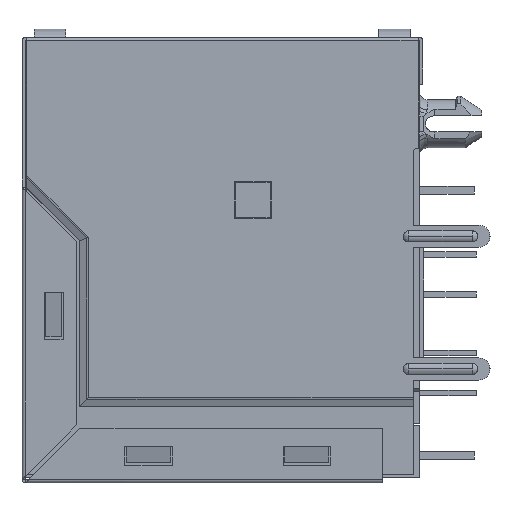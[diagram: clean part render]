
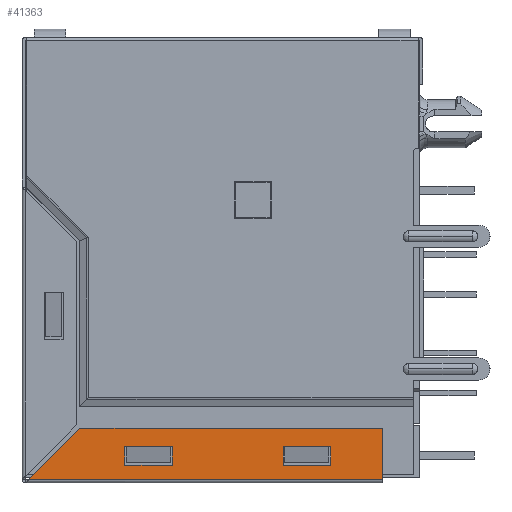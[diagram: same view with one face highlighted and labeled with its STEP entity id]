
A CAD part, left-side view. The second image highlights one B-rep face of the part: STEP entity #41363.
In plain terms, the highlighted planar face has unit normal (-1, 0, 0).
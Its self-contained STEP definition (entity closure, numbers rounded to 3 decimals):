
#149 = EDGE_CURVE ( 'NONE', #71271, #63621, #42202, .T. ) ;
#199 = EDGE_CURVE ( 'NONE', #31274, #15302, #2112, .T. ) ;
#1811 = EDGE_LOOP ( 'NONE', ( #43591, #2612, #13545, #4547 ) ) ;
#2112 = B_SPLINE_CURVE_WITH_KNOTS ( 'NONE', 1,
 ( #37321, #13007 ),
 .UNSPECIFIED., .F., .F.,
 ( 2, 2 ),
 ( 0., 1. ),
 .UNSPECIFIED. ) ;
#2612 = ORIENTED_EDGE ( 'NONE', *, *, #149, .T. ) ;
#3818 = CARTESIAN_POINT ( 'NONE',  ( -31.88, 6.165, -25.58 ) ) ;
#4150 = CARTESIAN_POINT ( 'NONE',  ( -31.88, 3.165, -25.58 ) ) ;
#4243 = CARTESIAN_POINT ( 'NONE',  ( -31.88, 6.165, -26.78 ) ) ;
#4261 = B_SPLINE_CURVE_WITH_KNOTS ( 'NONE', 1,
 ( #71911, #40936 ),
 .UNSPECIFIED., .F., .F.,
 ( 2, 2 ),
 ( 0., 1. ),
 .UNSPECIFIED. ) ;
#4446 = B_SPLINE_CURVE_WITH_KNOTS ( 'NONE', 1,
 ( #66529, #36102 ),
 .UNSPECIFIED., .F., .F.,
 ( 2, 2 ),
 ( 0., 1. ),
 .UNSPECIFIED. ) ;
#4547 = ORIENTED_EDGE ( 'NONE', *, *, #18581, .T. ) ;
#4903 = VECTOR ( 'NONE', #34564, 1000. ) ;
#9027 = CARTESIAN_POINT ( 'NONE',  ( -31.88, 9.005, -24.43 ) ) ;
#9712 = CARTESIAN_POINT ( 'NONE',  ( -31.88, 3.165, -26.78 ) ) ;
#10594 = EDGE_LOOP ( 'NONE', ( #33533, #55277, #71674, #60568 ) ) ;
#11064 = ORIENTED_EDGE ( 'NONE', *, *, #18309, .F. ) ;
#12041 = CARTESIAN_POINT ( 'NONE',  ( -31.88, 9.005, -24.43 ) ) ;
#12898 = CARTESIAN_POINT ( 'NONE',  ( -31.88, 6.165, -26.78 ) ) ;
#13007 = CARTESIAN_POINT ( 'NONE',  ( -31.88, 6.165, -25.58 ) ) ;
#13483 = VERTEX_POINT ( 'NONE', #12041 ) ;
#13545 = ORIENTED_EDGE ( 'NONE', *, *, #63434, .T. ) ;
#15302 = VERTEX_POINT ( 'NONE', #42465 ) ;
#15619 = CARTESIAN_POINT ( 'NONE',  ( -31.88, 1.055, -27.67 ) ) ;
#18309 = EDGE_CURVE ( 'NONE', #62407, #21727, #28934, .T. ) ;
#18581 = EDGE_CURVE ( 'NONE', #70747, #31402, #37221, .T. ) ;
#19591 = ORIENTED_EDGE ( 'NONE', *, *, #33564, .T. ) ;
#19681 = EDGE_CURVE ( 'NONE', #13483, #41862, #59765, .T. ) ;
#20091 = CARTESIAN_POINT ( 'NONE',  ( -31.88, -10.135, -24.43 ) ) ;
#21066 = CARTESIAN_POINT ( 'NONE',  ( -31.88, 12.245, -27.67 ) ) ;
#21727 = VERTEX_POINT ( 'NONE', #22345 ) ;
#22345 = CARTESIAN_POINT ( 'NONE',  ( -31.88, -10.135, -27.67 ) ) ;
#22449 = VERTEX_POINT ( 'NONE', #72924 ) ;
#28934 = B_SPLINE_CURVE_WITH_KNOTS ( 'NONE', 1,
 ( #64945, #34481 ),
 .UNSPECIFIED., .F., .F.,
 ( 2, 2 ),
 ( 0., 1. ),
 .UNSPECIFIED. ) ;
#31274 = VERTEX_POINT ( 'NONE', #12898 ) ;
#31402 = VERTEX_POINT ( 'NONE', #31573 ) ;
#31573 = CARTESIAN_POINT ( 'NONE',  ( -31.88, -6.835, -25.58 ) ) ;
#33135 = B_SPLINE_CURVE_WITH_KNOTS ( 'NONE', 1,
 ( #75967, #38621 ),
 .UNSPECIFIED., .F., .F.,
 ( 2, 2 ),
 ( 0., 1. ),
 .UNSPECIFIED. ) ;
#33533 = ORIENTED_EDGE ( 'NONE', *, *, #52172, .T. ) ;
#33564 = EDGE_CURVE ( 'NONE', #62407, #13483, #4446, .T. ) ;
#34140 = B_SPLINE_CURVE_WITH_KNOTS ( 'NONE', 1,
 ( #4150, #9712 ),
 .UNSPECIFIED., .F., .F.,
 ( 2, 2 ),
 ( 0., 1. ),
 .UNSPECIFIED. ) ;
#34481 = CARTESIAN_POINT ( 'NONE',  ( -31.88, -10.135, -27.67 ) ) ;
#34564 = DIRECTION ( 'NONE',  ( 0., -1., 0. ) ) ;
#36102 = CARTESIAN_POINT ( 'NONE',  ( -31.88, 9.005, -24.43 ) ) ;
#36530 = CARTESIAN_POINT ( 'NONE',  ( -31.88, 12.693, -27.79 ) ) ;
#37221 = B_SPLINE_CURVE_WITH_KNOTS ( 'NONE', 1,
 ( #63263, #50471 ),
 .UNSPECIFIED., .F., .F.,
 ( 2, 2 ),
 ( 0., 1. ),
 .UNSPECIFIED. ) ;
#37321 = CARTESIAN_POINT ( 'NONE',  ( -31.88, 6.165, -26.78 ) ) ;
#38582 = CARTESIAN_POINT ( 'NONE',  ( -31.88, 12.245, -27.67 ) ) ;
#38621 = CARTESIAN_POINT ( 'NONE',  ( -31.88, -3.835, -25.58 ) ) ;
#40632 = CARTESIAN_POINT ( 'NONE',  ( -31.88, 3.165, -25.58 ) ) ;
#40936 = CARTESIAN_POINT ( 'NONE',  ( -31.88, -6.835, -26.78 ) ) ;
#41363 = ADVANCED_FACE ( 'NONE', ( #69511, #48483, #62793 ), #73120, .T. ) ;
#41862 = VERTEX_POINT ( 'NONE', #38582 ) ;
#42202 = B_SPLINE_CURVE_WITH_KNOTS ( 'NONE', 1,
 ( #72594, #54186 ),
 .UNSPECIFIED., .F., .F.,
 ( 2, 2 ),
 ( 0., 1. ),
 .UNSPECIFIED. ) ;
#42398 = DIRECTION ( 'NONE',  ( -1., 0., 0. ) ) ;
#42465 = CARTESIAN_POINT ( 'NONE',  ( -31.88, 6.165, -25.58 ) ) ;
#43591 = ORIENTED_EDGE ( 'NONE', *, *, #75378, .T. ) ;
#44405 = VERTEX_POINT ( 'NONE', #64665 ) ;
#46406 = CARTESIAN_POINT ( 'NONE',  ( -31.88, 3.165, -26.78 ) ) ;
#48483 = FACE_BOUND ( 'NONE', #1811, .T. ) ;
#50471 = CARTESIAN_POINT ( 'NONE',  ( -31.88, -6.835, -25.58 ) ) ;
#52172 = EDGE_CURVE ( 'NONE', #44405, #22449, #34140, .T. ) ;
#52489 = ORIENTED_EDGE ( 'NONE', *, *, #63573, .T. ) ;
#53605 = LINE ( 'NONE', #15619, #4903 ) ;
#54186 = CARTESIAN_POINT ( 'NONE',  ( -31.88, -3.835, -26.78 ) ) ;
#55277 = ORIENTED_EDGE ( 'NONE', *, *, #58386, .T. ) ;
#55483 = DIRECTION ( 'NONE',  ( 0., -1., 0. ) ) ;
#56678 = B_SPLINE_CURVE_WITH_KNOTS ( 'NONE', 1,
 ( #46406, #4243 ),
 .UNSPECIFIED., .F., .F.,
 ( 2, 2 ),
 ( 0., 1. ),
 .UNSPECIFIED. ) ;
#58386 = EDGE_CURVE ( 'NONE', #22449, #31274, #56678, .T. ) ;
#59765 = B_SPLINE_CURVE_WITH_KNOTS ( 'NONE', 1,
 ( #9027, #21066 ),
 .UNSPECIFIED., .F., .F.,
 ( 2, 2 ),
 ( 0., 1. ),
 .UNSPECIFIED. ) ;
#60568 = ORIENTED_EDGE ( 'NONE', *, *, #65749, .T. ) ;
#61795 = ORIENTED_EDGE ( 'NONE', *, *, #19681, .T. ) ;
#62407 = VERTEX_POINT ( 'NONE', #20091 ) ;
#62793 = FACE_BOUND ( 'NONE', #10594, .T. ) ;
#63263 = CARTESIAN_POINT ( 'NONE',  ( -31.88, -3.835, -25.58 ) ) ;
#63434 = EDGE_CURVE ( 'NONE', #63621, #70747, #33135, .T. ) ;
#63573 = EDGE_CURVE ( 'NONE', #41862, #21727, #53605, .T. ) ;
#63621 = VERTEX_POINT ( 'NONE', #70090 ) ;
#64665 = CARTESIAN_POINT ( 'NONE',  ( -31.88, 3.165, -25.58 ) ) ;
#64945 = CARTESIAN_POINT ( 'NONE',  ( -31.88, -10.135, -24.43 ) ) ;
#65749 = EDGE_CURVE ( 'NONE', #15302, #44405, #74735, .T. ) ;
#66529 = CARTESIAN_POINT ( 'NONE',  ( -31.88, -10.135, -24.43 ) ) ;
#67607 = AXIS2_PLACEMENT_3D ( 'NONE', #36530, #42398, #55483 ) ;
#69511 = FACE_OUTER_BOUND ( 'NONE', #73060, .T. ) ;
#70090 = CARTESIAN_POINT ( 'NONE',  ( -31.88, -3.835, -26.78 ) ) ;
#70747 = VERTEX_POINT ( 'NONE', #73305 ) ;
#71271 = VERTEX_POINT ( 'NONE', #78035 ) ;
#71674 = ORIENTED_EDGE ( 'NONE', *, *, #199, .T. ) ;
#71911 = CARTESIAN_POINT ( 'NONE',  ( -31.88, -6.835, -25.58 ) ) ;
#72594 = CARTESIAN_POINT ( 'NONE',  ( -31.88, -6.835, -26.78 ) ) ;
#72924 = CARTESIAN_POINT ( 'NONE',  ( -31.88, 3.165, -26.78 ) ) ;
#73060 = EDGE_LOOP ( 'NONE', ( #11064, #19591, #61795, #52489 ) ) ;
#73120 = PLANE ( 'NONE',  #67607 ) ;
#73305 = CARTESIAN_POINT ( 'NONE',  ( -31.88, -3.835, -25.58 ) ) ;
#74735 = B_SPLINE_CURVE_WITH_KNOTS ( 'NONE', 1,
 ( #3818, #40632 ),
 .UNSPECIFIED., .F., .F.,
 ( 2, 2 ),
 ( 0., 1. ),
 .UNSPECIFIED. ) ;
#75378 = EDGE_CURVE ( 'NONE', #31402, #71271, #4261, .T. ) ;
#75967 = CARTESIAN_POINT ( 'NONE',  ( -31.88, -3.835, -26.78 ) ) ;
#78035 = CARTESIAN_POINT ( 'NONE',  ( -31.88, -6.835, -26.78 ) ) ;
